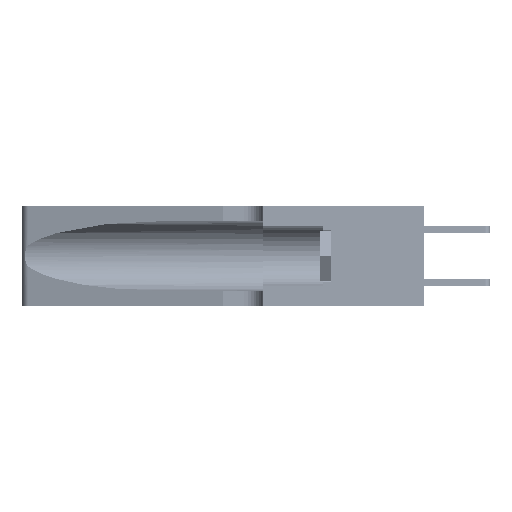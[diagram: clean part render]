
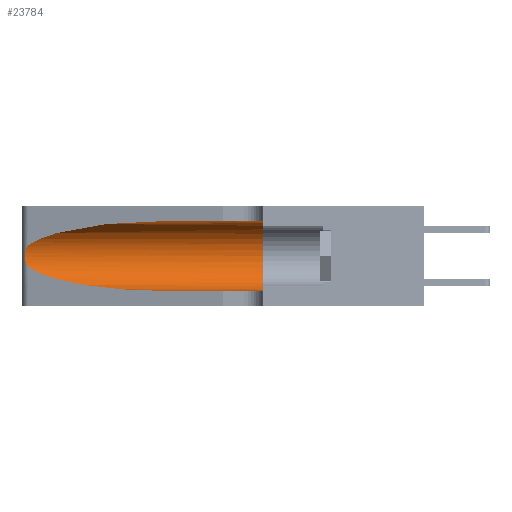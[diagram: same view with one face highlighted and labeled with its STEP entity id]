
A CAD part, left-side view. The second image highlights one B-rep face of the part: STEP entity #23784.
In plain terms, the highlighted cylindrical face has radius 3.308 mm (diameter 6.617 mm), a partial arc.
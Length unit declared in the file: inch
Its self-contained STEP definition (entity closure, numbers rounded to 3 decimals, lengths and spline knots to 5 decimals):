
#21 = CARTESIAN_POINT ( 'NONE',  ( 0.25639, 1.23184, 0.21858 ) ) ;
#253 = CYLINDRICAL_SURFACE ( 'NONE', #11518, 0.13025 ) ;
#984 = CARTESIAN_POINT ( 'NONE',  ( 0.2373, 1.15595, 0.28018 ) ) ;
#3907 = CARTESIAN_POINT ( 'NONE',  ( 0.26018, 1.23835, 0.19895 ) ) ;
#4649 = CARTESIAN_POINT ( 'NONE',  ( 0.1305, 0.72297, 0.05475 ) ) ;
#4815 = CARTESIAN_POINT ( 'NONE',  ( 0.25487, 1.22718, 0.14631 ) ) ;
#7387 = CIRCLE ( 'NONE', #50101, 0.13025 ) ;
#8508 = ORIENTED_EDGE ( 'NONE', *, *, #9660, .T. ) ;
#9240 = CARTESIAN_POINT ( 'NONE',  ( 0.18966, 0.96281, 0.31525 ) ) ;
#9433 = EDGE_LOOP ( 'NONE', ( #8508, #17988, #48965, #41532, #17400, #24652 ) ) ;
#9660 = EDGE_CURVE ( 'NONE', #13575, #39642, #10803, .T. ) ;
#10803 =( BOUNDED_CURVE ( )  B_SPLINE_CURVE ( 3, ( #41313, #9240, #984, #49404 ),
 .UNSPECIFIED., .F., .T. ) 
 B_SPLINE_CURVE_WITH_KNOTS ( ( 4, 4 ),
 ( 1.5708, 2.84003 ),
 .UNSPECIFIED. ) 
 CURVE ( )  GEOMETRIC_REPRESENTATION_ITEM ( )  RATIONAL_B_SPLINE_CURVE ( ( 1., 0.87, 0.87, 1. ) ) 
 REPRESENTATION_ITEM ( '' )  );
#11518 = AXIS2_PLACEMENT_3D ( 'NONE', #24384, #19840, #40182 ) ;
#12471 = CARTESIAN_POINT ( 'NONE',  ( 0.25639, 1.23186, 0.15144 ) ) ;
#13575 = VERTEX_POINT ( 'NONE', #41500 ) ;
#13718 = VECTOR ( 'NONE', #42909, 39.37008 ) ;
#14525 = CARTESIAN_POINT ( 'NONE',  ( 0.1305, 0.35, 0.05475 ) ) ;
#16109 = VERTEX_POINT ( 'NONE', #4815 ) ;
#16135 = CARTESIAN_POINT ( 'NONE',  ( 0.25856, 1.23593, 0.16098 ) ) ;
#16692 = DIRECTION ( 'NONE',  ( 0., -1., 0. ) ) ;
#17400 = ORIENTED_EDGE ( 'NONE', *, *, #33086, .F. ) ;
#17988 = ORIENTED_EDGE ( 'NONE', *, *, #44124, .T. ) ;
#18625 = CARTESIAN_POINT ( 'NONE',  ( 0.25487, 1.22718, 0.22369 ) ) ;
#19840 = DIRECTION ( 'NONE',  ( 0., -1., 0. ) ) ;
#20070 = CARTESIAN_POINT ( 'NONE',  ( 0.1305, 0.35, 0.185 ) ) ;
#20360 = CARTESIAN_POINT ( 'NONE',  ( 0.25555, 1.22993, 0.14849 ) ) ;
#20839 = VECTOR ( 'NONE', #16692, 39.37008 ) ;
#21885 = LINE ( 'NONE', #43429, #13718 ) ;
#22366 =( BOUNDED_CURVE ( )  B_SPLINE_CURVE ( 3, ( #39882, #44282, #48344, #4649 ),
 .UNSPECIFIED., .F., .T. ) 
 B_SPLINE_CURVE_WITH_KNOTS ( ( 4, 4 ),
 ( 3.44316, 4.71239 ),
 .UNSPECIFIED. ) 
 CURVE ( )  GEOMETRIC_REPRESENTATION_ITEM ( )  RATIONAL_B_SPLINE_CURVE ( ( 1., 0.87, 0.87, 1. ) ) 
 REPRESENTATION_ITEM ( '' )  );
#23784 = ADVANCED_FACE ( 'NONE', ( #30384 ), #253, .F. ) ;
#23871 = CARTESIAN_POINT ( 'NONE',  ( 0.25487, 1.22718, 0.22369 ) ) ;
#24384 = CARTESIAN_POINT ( 'NONE',  ( 0.1305, 1.61858, 0.185 ) ) ;
#24652 = ORIENTED_EDGE ( 'NONE', *, *, #37884, .F. ) ;
#26209 = EDGE_CURVE ( 'NONE', #16109, #31342, #22366, .T. ) ;
#27157 = VERTEX_POINT ( 'NONE', #14525 ) ;
#27792 = DIRECTION ( 'NONE',  ( 0., 1., 0. ) ) ;
#28065 = CARTESIAN_POINT ( 'NONE',  ( 0.26075, 1.23896, 0.19203 ) ) ;
#28188 = CARTESIAN_POINT ( 'NONE',  ( 0.1305, 0.72297, 0.05475 ) ) ;
#30384 = FACE_OUTER_BOUND ( 'NONE', #9433, .T. ) ;
#31342 = VERTEX_POINT ( 'NONE', #28188 ) ;
#32297 = CARTESIAN_POINT ( 'NONE',  ( 0.1305, 0.35, 0.31525 ) ) ;
#33086 = EDGE_CURVE ( 'NONE', #41765, #27157, #7387, .T. ) ;
#36299 = EDGE_CURVE ( 'NONE', #31342, #27157, #36496, .T. ) ;
#36496 = LINE ( 'NONE', #45312, #20839 ) ;
#37884 = EDGE_CURVE ( 'NONE', #13575, #41765, #21885, .T. ) ;
#39642 = VERTEX_POINT ( 'NONE', #18625 ) ;
#39664 = CARTESIAN_POINT ( 'NONE',  ( 0.26017, 1.23833, 0.17102 ) ) ;
#39730 = DIRECTION ( 'NONE',  ( 0., 0., 1. ) ) ;
#39882 = CARTESIAN_POINT ( 'NONE',  ( 0.25487, 1.22718, 0.14631 ) ) ;
#40175 = CARTESIAN_POINT ( 'NONE',  ( 0.26075, 1.23896, 0.178 ) ) ;
#40182 = DIRECTION ( 'NONE',  ( 0., 0., -1. ) ) ;
#41313 = CARTESIAN_POINT ( 'NONE',  ( 0.1305, 0.72297, 0.31525 ) ) ;
#41500 = CARTESIAN_POINT ( 'NONE',  ( 0.1305, 0.72297, 0.31525 ) ) ;
#41532 = ORIENTED_EDGE ( 'NONE', *, *, #36299, .T. ) ;
#41765 = VERTEX_POINT ( 'NONE', #32297 ) ;
#42909 = DIRECTION ( 'NONE',  ( 0., -1., 0. ) ) ;
#43429 = CARTESIAN_POINT ( 'NONE',  ( 0.1305, 1.61858, 0.31525 ) ) ;
#43536 = CARTESIAN_POINT ( 'NONE',  ( 0.25555, 1.22994, 0.2215 ) ) ;
#44124 = EDGE_CURVE ( 'NONE', #39642, #16109, #50376, .T. ) ;
#44282 = CARTESIAN_POINT ( 'NONE',  ( 0.2373, 1.15595, 0.08982 ) ) ;
#45090 = CARTESIAN_POINT ( 'NONE',  ( 0.25487, 1.22718, 0.14631 ) ) ;
#45312 = CARTESIAN_POINT ( 'NONE',  ( 0.1305, 1.61858, 0.05475 ) ) ;
#47609 = CARTESIAN_POINT ( 'NONE',  ( 0.25787, 1.23484, 0.2124 ) ) ;
#48281 = CARTESIAN_POINT ( 'NONE',  ( 0.25789, 1.23486, 0.15765 ) ) ;
#48344 = CARTESIAN_POINT ( 'NONE',  ( 0.18966, 0.96281, 0.05475 ) ) ;
#48965 = ORIENTED_EDGE ( 'NONE', *, *, #26209, .T. ) ;
#49404 = CARTESIAN_POINT ( 'NONE',  ( 0.25487, 1.22718, 0.22369 ) ) ;
#50101 = AXIS2_PLACEMENT_3D ( 'NONE', #20070, #27792, #39730 ) ;
#50376 = B_SPLINE_CURVE_WITH_KNOTS ( 'NONE', 3,
 ( #23871, #43536, #21, #47609, #51964, #3907, #28065, #40175, #39664, #16135, #48281, #12471, #20360, #45090 ),
 .UNSPECIFIED., .F., .F.,
 ( 4, 2, 2, 2, 2, 2, 4 ),
 ( 0., 0.00027, 0.00053, 0.00107, 0.0016, 0.00187, 0.00214 ),
 .UNSPECIFIED. ) ;
#51964 = CARTESIAN_POINT ( 'NONE',  ( 0.25854, 1.2359, 0.20912 ) ) ;
